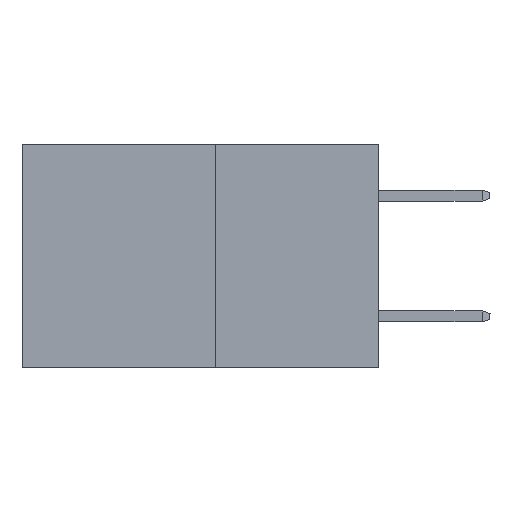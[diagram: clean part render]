
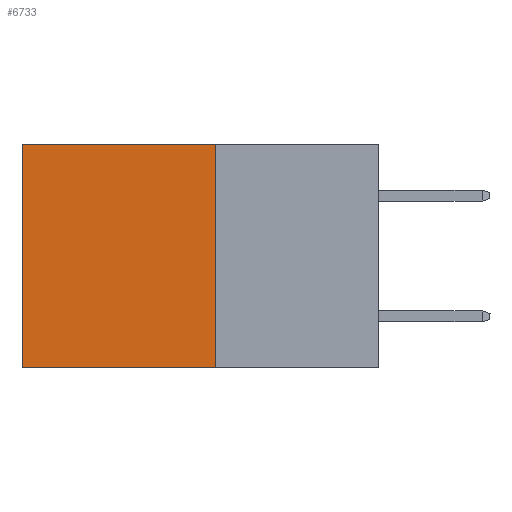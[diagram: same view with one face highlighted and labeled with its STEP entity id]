
A CAD part, left-side view. The second image highlights one B-rep face of the part: STEP entity #6733.
In plain terms, the highlighted planar face has unit normal (-1, 0, 0).
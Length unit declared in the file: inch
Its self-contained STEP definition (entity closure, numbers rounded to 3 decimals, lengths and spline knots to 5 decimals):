
#262 = CARTESIAN_POINT ( 'NONE',  ( 0.277, 0.59, 0. ) ) ;
#362 = AXIS2_PLACEMENT_3D ( 'NONE', #10861, #8452, #3372 ) ;
#792 = ORIENTED_EDGE ( 'NONE', *, *, #12332, .F. ) ;
#1096 = ORIENTED_EDGE ( 'NONE', *, *, #3259, .T. ) ;
#1272 = LINE ( 'NONE', #8995, #6355 ) ;
#2107 = LINE ( 'NONE', #6597, #12961 ) ;
#2274 = EDGE_CURVE ( 'NONE', #5168, #12756, #11134, .T. ) ;
#2511 = ORIENTED_EDGE ( 'NONE', *, *, #2274, .T. ) ;
#2758 = VECTOR ( 'NONE', #6434, 39.37008 ) ;
#3259 = EDGE_CURVE ( 'NONE', #9315, #5168, #8959, .T. ) ;
#3372 = DIRECTION ( 'NONE',  ( 0., 0., -1. ) ) ;
#4676 = CARTESIAN_POINT ( 'NONE',  ( 0.277, 0.59, -0.37 ) ) ;
#5168 = VERTEX_POINT ( 'NONE', #262 ) ;
#5349 = PLANE ( 'NONE',  #362 ) ;
#5935 = EDGE_LOOP ( 'NONE', ( #2511, #792, #11657, #1096 ) ) ;
#6355 = VECTOR ( 'NONE', #9995, 39.37008 ) ;
#6434 = DIRECTION ( 'NONE',  ( 0., 1., 0. ) ) ;
#6597 = CARTESIAN_POINT ( 'NONE',  ( 0.277, 0.27, -0.37 ) ) ;
#6711 = CARTESIAN_POINT ( 'NONE',  ( 0.277, 0.27, -0.37 ) ) ;
#6733 = ADVANCED_FACE ( 'NONE', ( #6977 ), #5349, .F. ) ;
#6977 = FACE_OUTER_BOUND ( 'NONE', #5935, .T. ) ;
#7285 = VERTEX_POINT ( 'NONE', #6711 ) ;
#7458 = CARTESIAN_POINT ( 'NONE',  ( 0.277, 0.59, -0.37 ) ) ;
#7643 = DIRECTION ( 'NONE',  ( 0., 0., -1. ) ) ;
#8452 = DIRECTION ( 'NONE',  ( 1., 0., 0. ) ) ;
#8781 = VECTOR ( 'NONE', #7643, 39.37008 ) ;
#8959 = LINE ( 'NONE', #9459, #2758 ) ;
#8995 = CARTESIAN_POINT ( 'NONE',  ( 0.277, 0.27, -0.37 ) ) ;
#9315 = VERTEX_POINT ( 'NONE', #12426 ) ;
#9459 = CARTESIAN_POINT ( 'NONE',  ( 0.277, 0.27, 0. ) ) ;
#9843 = EDGE_CURVE ( 'NONE', #9315, #7285, #2107, .T. ) ;
#9995 = DIRECTION ( 'NONE',  ( 0., 1., 0. ) ) ;
#10861 = CARTESIAN_POINT ( 'NONE',  ( 0.277, 0.27, -0.37 ) ) ;
#10905 = DIRECTION ( 'NONE',  ( 0., 0., -1. ) ) ;
#11134 = LINE ( 'NONE', #7458, #8781 ) ;
#11657 = ORIENTED_EDGE ( 'NONE', *, *, #9843, .F. ) ;
#12332 = EDGE_CURVE ( 'NONE', #7285, #12756, #1272, .T. ) ;
#12426 = CARTESIAN_POINT ( 'NONE',  ( 0.277, 0.27, 0. ) ) ;
#12756 = VERTEX_POINT ( 'NONE', #4676 ) ;
#12961 = VECTOR ( 'NONE', #10905, 39.37008 ) ;
